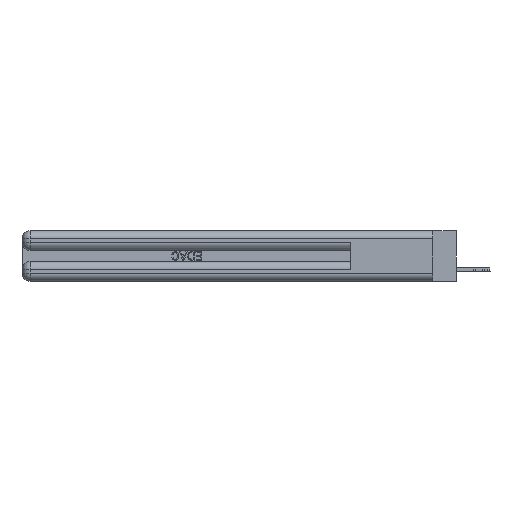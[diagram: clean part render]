
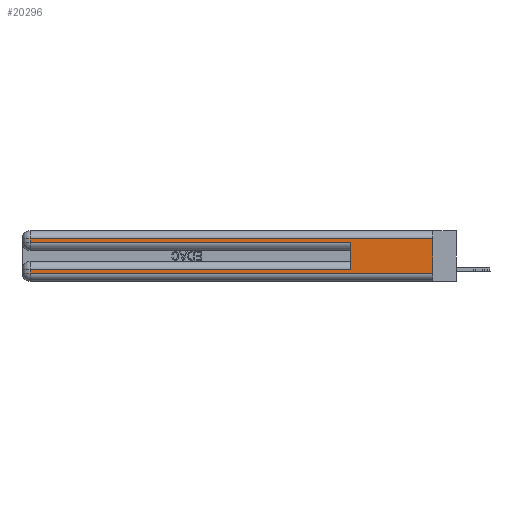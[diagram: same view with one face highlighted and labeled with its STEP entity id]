
A CAD part, left-side view. The second image highlights one B-rep face of the part: STEP entity #20296.
In plain terms, the highlighted planar face has unit normal (-1, 0, 0).
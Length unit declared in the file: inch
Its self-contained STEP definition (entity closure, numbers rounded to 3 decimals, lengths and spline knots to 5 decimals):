
#129 = CARTESIAN_POINT ( 'NONE',  ( 0., 0., 0.285 ) ) ;
#891 = VERTEX_POINT ( 'NONE', #15636 ) ;
#2325 = CARTESIAN_POINT ( 'NONE',  ( 0., 2.94, 0.31 ) ) ;
#2965 = EDGE_CURVE ( 'NONE', #34785, #891, #48000, .T. ) ;
#3176 = DIRECTION ( 'NONE',  ( 0., 1., 0. ) ) ;
#3667 = DIRECTION ( 'NONE',  ( 0., 0., 1. ) ) ;
#3767 = LINE ( 'NONE', #45602, #30485 ) ;
#5698 = VERTEX_POINT ( 'NONE', #26148 ) ;
#8532 = VECTOR ( 'NONE', #10850, 39.37008 ) ;
#9227 = FACE_OUTER_BOUND ( 'NONE', #41453, .T. ) ;
#9627 = EDGE_CURVE ( 'NONE', #23586, #891, #39367, .T. ) ;
#10328 = ORIENTED_EDGE ( 'NONE', *, *, #13912, .T. ) ;
#10377 = CARTESIAN_POINT ( 'NONE',  ( 0., 2.94, 0.06 ) ) ;
#10850 = DIRECTION ( 'NONE',  ( 0., 1., 0. ) ) ;
#11022 = EDGE_CURVE ( 'NONE', #50399, #5698, #19923, .T. ) ;
#11677 = DIRECTION ( 'NONE',  ( 0., 0., -1. ) ) ;
#12093 = ORIENTED_EDGE ( 'NONE', *, *, #9627, .T. ) ;
#12793 = ORIENTED_EDGE ( 'NONE', *, *, #11022, .T. ) ;
#13912 = EDGE_CURVE ( 'NONE', #36812, #23453, #48207, .T. ) ;
#14549 = CARTESIAN_POINT ( 'NONE',  ( 0., 2.94, 0.37 ) ) ;
#15636 = CARTESIAN_POINT ( 'NONE',  ( 0., 0., 0.06 ) ) ;
#15800 = CARTESIAN_POINT ( 'NONE',  ( 0., 0., 0.06 ) ) ;
#15856 = ORIENTED_EDGE ( 'NONE', *, *, #22077, .T. ) ;
#17649 = LINE ( 'NONE', #25198, #44336 ) ;
#18265 = EDGE_CURVE ( 'NONE', #5698, #23586, #53576, .T. ) ;
#18637 = VECTOR ( 'NONE', #40548, 39.37008 ) ;
#19923 = LINE ( 'NONE', #36449, #8532 ) ;
#19977 = ORIENTED_EDGE ( 'NONE', *, *, #18265, .T. ) ;
#20028 = CARTESIAN_POINT ( 'NONE',  ( 0., 2.94, 0.285 ) ) ;
#20296 = ADVANCED_FACE ( 'NONE', ( #9227 ), #51955, .F. ) ;
#21803 = DIRECTION ( 'NONE',  ( 0., -1., 0. ) ) ;
#22077 = EDGE_CURVE ( 'NONE', #34785, #36812, #3767, .T. ) ;
#23453 = VERTEX_POINT ( 'NONE', #20028 ) ;
#23586 = VERTEX_POINT ( 'NONE', #10377 ) ;
#23952 = CARTESIAN_POINT ( 'NONE',  ( 0., 2.94, 0.37 ) ) ;
#25007 = ORIENTED_EDGE ( 'NONE', *, *, #41306, .F. ) ;
#25198 = CARTESIAN_POINT ( 'NONE',  ( 0., 0.6, 0.145 ) ) ;
#26148 = CARTESIAN_POINT ( 'NONE',  ( 0., 2.94, 0.085 ) ) ;
#26818 = DIRECTION ( 'NONE',  ( 1., 0., 0. ) ) ;
#28280 = DIRECTION ( 'NONE',  ( 0., -1., 0. ) ) ;
#29173 = CARTESIAN_POINT ( 'NONE',  ( 0., 0., 0.31 ) ) ;
#29605 = CARTESIAN_POINT ( 'NONE',  ( 0., 0., 0.37 ) ) ;
#30485 = VECTOR ( 'NONE', #3176, 39.37008 ) ;
#32965 = DIRECTION ( 'NONE',  ( 0., 0., -1. ) ) ;
#34785 = VERTEX_POINT ( 'NONE', #29173 ) ;
#34790 = VECTOR ( 'NONE', #21803, 39.37008 ) ;
#36449 = CARTESIAN_POINT ( 'NONE',  ( 0., 0., 0.085 ) ) ;
#36812 = VERTEX_POINT ( 'NONE', #2325 ) ;
#36821 = ORIENTED_EDGE ( 'NONE', *, *, #48674, .T. ) ;
#38170 = VECTOR ( 'NONE', #28280, 39.37008 ) ;
#39367 = LINE ( 'NONE', #15800, #38170 ) ;
#39387 = LINE ( 'NONE', #129, #34790 ) ;
#40548 = DIRECTION ( 'NONE',  ( 0., 0., -1. ) ) ;
#41306 = EDGE_CURVE ( 'NONE', #50399, #46622, #17649, .T. ) ;
#41453 = EDGE_LOOP ( 'NONE', ( #44539, #15856, #10328, #36821, #25007, #12793, #19977, #12093 ) ) ;
#42284 = VECTOR ( 'NONE', #32965, 39.37008 ) ;
#44193 = AXIS2_PLACEMENT_3D ( 'NONE', #29605, #26818, #49008 ) ;
#44336 = VECTOR ( 'NONE', #3667, 39.37008 ) ;
#44539 = ORIENTED_EDGE ( 'NONE', *, *, #2965, .F. ) ;
#45602 = CARTESIAN_POINT ( 'NONE',  ( 0., 0., 0.31 ) ) ;
#46622 = VERTEX_POINT ( 'NONE', #49653 ) ;
#46986 = VECTOR ( 'NONE', #11677, 39.37008 ) ;
#48000 = LINE ( 'NONE', #53710, #18637 ) ;
#48207 = LINE ( 'NONE', #14549, #46986 ) ;
#48674 = EDGE_CURVE ( 'NONE', #23453, #46622, #39387, .T. ) ;
#49008 = DIRECTION ( 'NONE',  ( 0., 0., -1. ) ) ;
#49653 = CARTESIAN_POINT ( 'NONE',  ( 0., 0.6, 0.285 ) ) ;
#50399 = VERTEX_POINT ( 'NONE', #51413 ) ;
#51413 = CARTESIAN_POINT ( 'NONE',  ( 0., 0.6, 0.085 ) ) ;
#51955 = PLANE ( 'NONE',  #44193 ) ;
#53576 = LINE ( 'NONE', #23952, #42284 ) ;
#53710 = CARTESIAN_POINT ( 'NONE',  ( 0., 0., 0.37 ) ) ;
